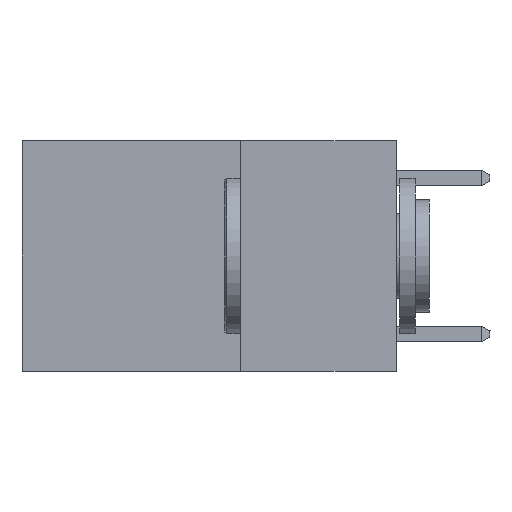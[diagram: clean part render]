
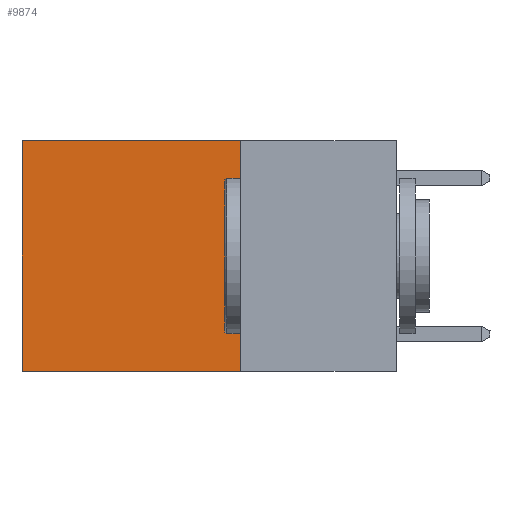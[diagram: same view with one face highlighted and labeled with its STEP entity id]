
A CAD part, left-side view. The second image highlights one B-rep face of the part: STEP entity #9874.
In plain terms, the highlighted planar face has unit normal (-1, 0, 0).
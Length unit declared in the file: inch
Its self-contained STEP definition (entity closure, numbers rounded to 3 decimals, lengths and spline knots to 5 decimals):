
#505 = VECTOR ( 'NONE', #5845, 39.37008 ) ;
#933 = VERTEX_POINT ( 'NONE', #5328 ) ;
#1417 = EDGE_CURVE ( 'NONE', #933, #9001, #17501, .T. ) ;
#1776 = VECTOR ( 'NONE', #22598, 39.37008 ) ;
#3296 = EDGE_CURVE ( 'NONE', #12597, #18238, #8182, .T. ) ;
#5328 = CARTESIAN_POINT ( 'NONE',  ( 0.2625, 0.25, 0. ) ) ;
#5477 = CARTESIAN_POINT ( 'NONE',  ( 0.2625, 0.6, -0.37 ) ) ;
#5845 = DIRECTION ( 'NONE',  ( 0., 0., -1. ) ) ;
#6387 = CARTESIAN_POINT ( 'NONE',  ( 0.2625, 0.25, 0. ) ) ;
#8093 = VECTOR ( 'NONE', #11276, 39.37008 ) ;
#8182 = LINE ( 'NONE', #21666, #8093 ) ;
#8335 = ORIENTED_EDGE ( 'NONE', *, *, #17019, .T. ) ;
#8521 = DIRECTION ( 'NONE',  ( 1., 0., 0. ) ) ;
#9001 = VERTEX_POINT ( 'NONE', #23870 ) ;
#9874 = ADVANCED_FACE ( 'NONE', ( #16466 ), #16906, .F. ) ;
#10103 = CARTESIAN_POINT ( 'NONE',  ( 0.2625, 0.6, 0. ) ) ;
#11276 = DIRECTION ( 'NONE',  ( 0., 1., 0. ) ) ;
#12597 = VERTEX_POINT ( 'NONE', #25032 ) ;
#14097 = ORIENTED_EDGE ( 'NONE', *, *, #21607, .F. ) ;
#15211 = DIRECTION ( 'NONE',  ( 0., 1., 0. ) ) ;
#16466 = FACE_OUTER_BOUND ( 'NONE', #25839, .T. ) ;
#16906 = PLANE ( 'NONE',  #22037 ) ;
#17019 = EDGE_CURVE ( 'NONE', #9001, #18238, #23633, .T. ) ;
#17245 = CARTESIAN_POINT ( 'NONE',  ( 0.2625, 0.25, 0. ) ) ;
#17322 = VECTOR ( 'NONE', #15211, 39.37008 ) ;
#17501 = LINE ( 'NONE', #17245, #17322 ) ;
#18238 = VERTEX_POINT ( 'NONE', #5477 ) ;
#18727 = LINE ( 'NONE', #20497, #1776 ) ;
#20007 = ORIENTED_EDGE ( 'NONE', *, *, #1417, .T. ) ;
#20497 = CARTESIAN_POINT ( 'NONE',  ( 0.2625, 0.25, 0. ) ) ;
#20820 = ORIENTED_EDGE ( 'NONE', *, *, #3296, .F. ) ;
#21607 = EDGE_CURVE ( 'NONE', #933, #12597, #18727, .T. ) ;
#21666 = CARTESIAN_POINT ( 'NONE',  ( 0.2625, 0.25, -0.37 ) ) ;
#22037 = AXIS2_PLACEMENT_3D ( 'NONE', #6387, #8521, #23102 ) ;
#22598 = DIRECTION ( 'NONE',  ( 0., 0., -1. ) ) ;
#23102 = DIRECTION ( 'NONE',  ( 0., 0., -1. ) ) ;
#23633 = LINE ( 'NONE', #10103, #505 ) ;
#23870 = CARTESIAN_POINT ( 'NONE',  ( 0.2625, 0.6, 0. ) ) ;
#25032 = CARTESIAN_POINT ( 'NONE',  ( 0.2625, 0.25, -0.37 ) ) ;
#25839 = EDGE_LOOP ( 'NONE', ( #8335, #20820, #14097, #20007 ) ) ;
